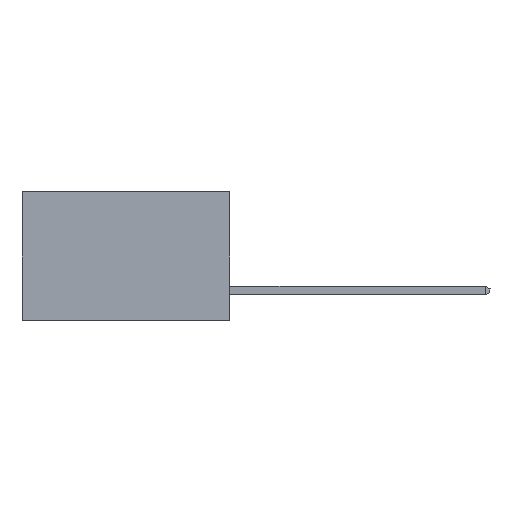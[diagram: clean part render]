
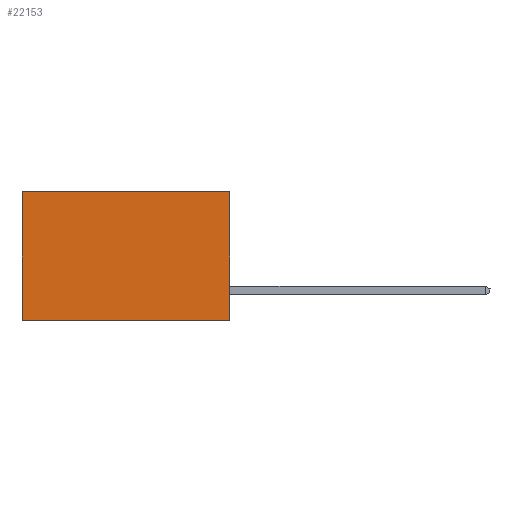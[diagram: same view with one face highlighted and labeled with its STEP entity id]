
A CAD part, left-side view. The second image highlights one B-rep face of the part: STEP entity #22153.
In plain terms, the highlighted planar face has unit normal (-1, 0, 0).
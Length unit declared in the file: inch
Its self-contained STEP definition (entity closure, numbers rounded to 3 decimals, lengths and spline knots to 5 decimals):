
#1061 = LINE ( 'NONE', #7976, #18277 ) ;
#2648 = LINE ( 'NONE', #9563, #17820 ) ;
#4865 = EDGE_CURVE ( 'NONE', #10583, #15812, #2648, .T. ) ;
#5158 = VECTOR ( 'NONE', #6522, 39.37008 ) ;
#6522 = DIRECTION ( 'NONE',  ( 0., 0., -1. ) ) ;
#7609 = VECTOR ( 'NONE', #9194, 39.37008 ) ;
#7976 = CARTESIAN_POINT ( 'NONE',  ( 0.2615, 0., 0. ) ) ;
#8065 = DIRECTION ( 'NONE',  ( 0., 0., -1. ) ) ;
#9011 = ORIENTED_EDGE ( 'NONE', *, *, #19191, .T. ) ;
#9194 = DIRECTION ( 'NONE',  ( 0., 0., -1. ) ) ;
#9563 = CARTESIAN_POINT ( 'NONE',  ( 0.2615, 0., -0.37 ) ) ;
#9987 = CARTESIAN_POINT ( 'NONE',  ( 0.2615, 0., -0.37 ) ) ;
#10508 = EDGE_CURVE ( 'NONE', #10570, #15142, #1061, .T. ) ;
#10570 = VERTEX_POINT ( 'NONE', #11567 ) ;
#10583 = VERTEX_POINT ( 'NONE', #9987 ) ;
#10981 = LINE ( 'NONE', #17770, #7609 ) ;
#11277 = CARTESIAN_POINT ( 'NONE',  ( 0.2615, 0.6, -0.37 ) ) ;
#11546 = PLANE ( 'NONE',  #15067 ) ;
#11567 = CARTESIAN_POINT ( 'NONE',  ( 0.2615, 0., 0. ) ) ;
#13130 = FACE_OUTER_BOUND ( 'NONE', #18450, .T. ) ;
#14462 = ORIENTED_EDGE ( 'NONE', *, *, #16939, .F. ) ;
#14763 = DIRECTION ( 'NONE',  ( 0., 1., 0. ) ) ;
#14918 = CARTESIAN_POINT ( 'NONE',  ( 0.2615, 0.6, 0. ) ) ;
#15067 = AXIS2_PLACEMENT_3D ( 'NONE', #21836, #19925, #8065 ) ;
#15142 = VERTEX_POINT ( 'NONE', #14918 ) ;
#15812 = VERTEX_POINT ( 'NONE', #22154 ) ;
#16939 = EDGE_CURVE ( 'NONE', #10570, #10583, #10981, .T. ) ;
#17770 = CARTESIAN_POINT ( 'NONE',  ( 0.2615, 0., -0.37 ) ) ;
#17820 = VECTOR ( 'NONE', #14763, 39.37008 ) ;
#18277 = VECTOR ( 'NONE', #20385, 39.37008 ) ;
#18450 = EDGE_LOOP ( 'NONE', ( #9011, #20847, #14462, #19280 ) ) ;
#19191 = EDGE_CURVE ( 'NONE', #15142, #15812, #22333, .T. ) ;
#19280 = ORIENTED_EDGE ( 'NONE', *, *, #10508, .T. ) ;
#19925 = DIRECTION ( 'NONE',  ( 1., 0., 0. ) ) ;
#20385 = DIRECTION ( 'NONE',  ( 0., 1., 0. ) ) ;
#20847 = ORIENTED_EDGE ( 'NONE', *, *, #4865, .F. ) ;
#21836 = CARTESIAN_POINT ( 'NONE',  ( 0.2615, 0., -0.37 ) ) ;
#22153 = ADVANCED_FACE ( 'NONE', ( #13130 ), #11546, .F. ) ;
#22154 = CARTESIAN_POINT ( 'NONE',  ( 0.2615, 0.6, -0.37 ) ) ;
#22333 = LINE ( 'NONE', #11277, #5158 ) ;
